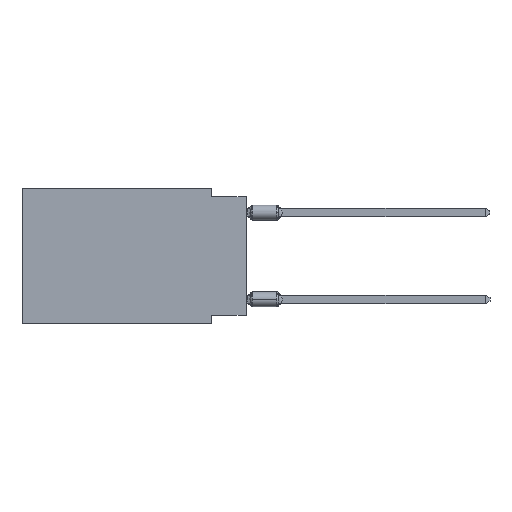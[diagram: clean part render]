
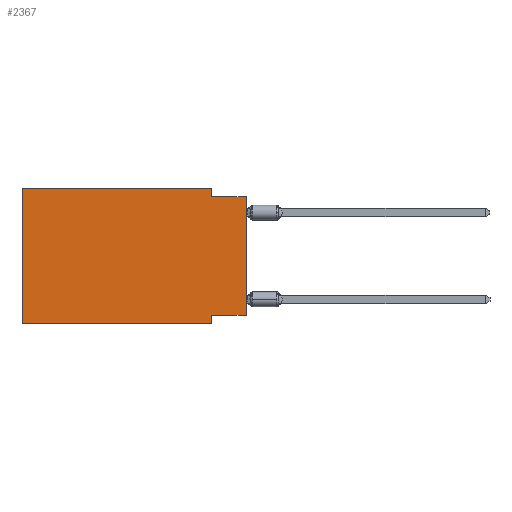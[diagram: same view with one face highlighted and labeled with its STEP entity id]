
A CAD part, left-side view. The second image highlights one B-rep face of the part: STEP entity #2367.
In plain terms, the highlighted planar face has unit normal (-1, 0, 0).
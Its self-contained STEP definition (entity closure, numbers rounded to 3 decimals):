
#89 = EDGE_CURVE ( 'NONE', #15713, #12112, #947, .T. ) ;
#238 = EDGE_CURVE ( 'NONE', #4727, #10262, #4256, .T. ) ;
#688 = CARTESIAN_POINT ( 'NONE',  ( 0., 16.383, 0. ) ) ;
#947 = LINE ( 'NONE', #9942, #10382 ) ;
#1034 = VECTOR ( 'NONE', #8260, 1000. ) ;
#1273 = ORIENTED_EDGE ( 'NONE', *, *, #17864, .T. ) ;
#1464 = ORIENTED_EDGE ( 'NONE', *, *, #3667, .F. ) ;
#1803 = CARTESIAN_POINT ( 'NONE',  ( 0., 2.54, 0. ) ) ;
#2102 = CARTESIAN_POINT ( 'NONE',  ( 0., 0., -9.271 ) ) ;
#2367 = ADVANCED_FACE ( 'NONE', ( #8651 ), #13293, .F. ) ;
#2559 = CARTESIAN_POINT ( 'NONE',  ( 0., 2.54, -9.271 ) ) ;
#2684 = CARTESIAN_POINT ( 'NONE',  ( 0., 16.383, 0. ) ) ;
#2844 = DIRECTION ( 'NONE',  ( 0., -1., 0. ) ) ;
#3001 = ORIENTED_EDGE ( 'NONE', *, *, #7586, .F. ) ;
#3318 = CARTESIAN_POINT ( 'NONE',  ( 0., 0., -0.635 ) ) ;
#3667 = EDGE_CURVE ( 'NONE', #5158, #12112, #11979, .T. ) ;
#4256 = LINE ( 'NONE', #10426, #6172 ) ;
#4424 = VECTOR ( 'NONE', #18117, 1000. ) ;
#4549 = VERTEX_POINT ( 'NONE', #17145 ) ;
#4727 = VERTEX_POINT ( 'NONE', #2684 ) ;
#5158 = VERTEX_POINT ( 'NONE', #2559 ) ;
#5600 = CARTESIAN_POINT ( 'NONE',  ( 0., 0., 0. ) ) ;
#6172 = VECTOR ( 'NONE', #2844, 1000. ) ;
#6550 = CARTESIAN_POINT ( 'NONE',  ( 0., 2.54, -0.635 ) ) ;
#6837 = DIRECTION ( 'NONE',  ( 0., 0., -1. ) ) ;
#7539 = ORIENTED_EDGE ( 'NONE', *, *, #10257, .F. ) ;
#7586 = EDGE_CURVE ( 'NONE', #8470, #5158, #14320, .T. ) ;
#8260 = DIRECTION ( 'NONE',  ( 0., 1., 0. ) ) ;
#8309 = VECTOR ( 'NONE', #13001, 1000. ) ;
#8347 = LINE ( 'NONE', #17638, #8309 ) ;
#8470 = VERTEX_POINT ( 'NONE', #12328 ) ;
#8651 = FACE_OUTER_BOUND ( 'NONE', #12593, .T. ) ;
#9115 = ORIENTED_EDGE ( 'NONE', *, *, #238, .F. ) ;
#9942 = CARTESIAN_POINT ( 'NONE',  ( 0., 16.383, -9.906 ) ) ;
#10257 = EDGE_CURVE ( 'NONE', #10262, #11616, #15637, .T. ) ;
#10262 = VERTEX_POINT ( 'NONE', #17460 ) ;
#10382 = VECTOR ( 'NONE', #19424, 1000. ) ;
#10426 = CARTESIAN_POINT ( 'NONE',  ( 0., 16.383, 0. ) ) ;
#11616 = VERTEX_POINT ( 'NONE', #6550 ) ;
#11670 = EDGE_CURVE ( 'NONE', #11616, #4549, #19072, .T. ) ;
#11979 = LINE ( 'NONE', #12173, #17750 ) ;
#12112 = VERTEX_POINT ( 'NONE', #15368 ) ;
#12173 = CARTESIAN_POINT ( 'NONE',  ( 0., 2.54, -9.906 ) ) ;
#12328 = CARTESIAN_POINT ( 'NONE',  ( 0., 0., -9.271 ) ) ;
#12593 = EDGE_LOOP ( 'NONE', ( #1273, #13040, #7539, #9115, #14907, #19169, #1464, #3001 ) ) ;
#12611 = DIRECTION ( 'NONE',  ( 0., -1., 0. ) ) ;
#13001 = DIRECTION ( 'NONE',  ( 0., 0., 1. ) ) ;
#13040 = ORIENTED_EDGE ( 'NONE', *, *, #11670, .F. ) ;
#13293 = PLANE ( 'NONE',  #16111 ) ;
#13409 = EDGE_CURVE ( 'NONE', #15713, #4727, #8347, .T. ) ;
#14320 = LINE ( 'NONE', #2102, #1034 ) ;
#14907 = ORIENTED_EDGE ( 'NONE', *, *, #13409, .F. ) ;
#14986 = LINE ( 'NONE', #5600, #4424 ) ;
#15368 = CARTESIAN_POINT ( 'NONE',  ( 0., 2.54, -9.906 ) ) ;
#15554 = CARTESIAN_POINT ( 'NONE',  ( 0., 16.383, -9.906 ) ) ;
#15637 = LINE ( 'NONE', #1803, #19375 ) ;
#15713 = VERTEX_POINT ( 'NONE', #15554 ) ;
#15810 = VECTOR ( 'NONE', #12611, 1000. ) ;
#16111 = AXIS2_PLACEMENT_3D ( 'NONE', #688, #17646, #6837 ) ;
#17145 = CARTESIAN_POINT ( 'NONE',  ( 0., 0., -0.635 ) ) ;
#17460 = CARTESIAN_POINT ( 'NONE',  ( 0., 2.54, 0. ) ) ;
#17638 = CARTESIAN_POINT ( 'NONE',  ( 0., 16.383, 0. ) ) ;
#17646 = DIRECTION ( 'NONE',  ( 1., 0., 0. ) ) ;
#17750 = VECTOR ( 'NONE', #19754, 1000. ) ;
#17864 = EDGE_CURVE ( 'NONE', #8470, #4549, #14986, .T. ) ;
#18117 = DIRECTION ( 'NONE',  ( 0., 0., 1. ) ) ;
#18861 = DIRECTION ( 'NONE',  ( 0., 0., -1. ) ) ;
#19072 = LINE ( 'NONE', #3318, #15810 ) ;
#19169 = ORIENTED_EDGE ( 'NONE', *, *, #89, .T. ) ;
#19375 = VECTOR ( 'NONE', #18861, 1000. ) ;
#19424 = DIRECTION ( 'NONE',  ( 0., -1., 0. ) ) ;
#19754 = DIRECTION ( 'NONE',  ( 0., 0., -1. ) ) ;
